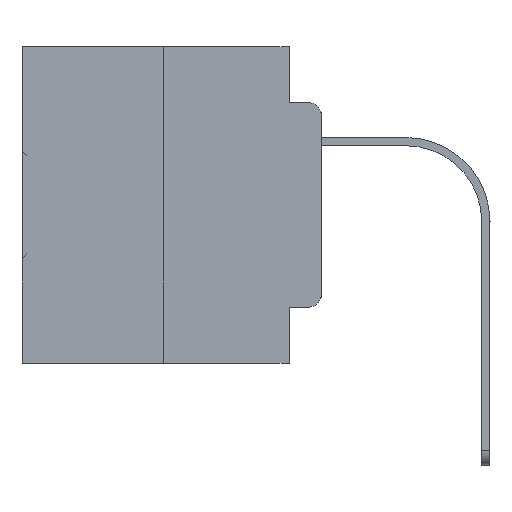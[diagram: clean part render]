
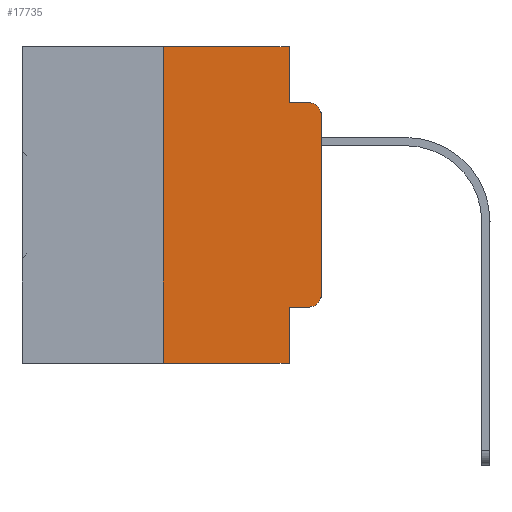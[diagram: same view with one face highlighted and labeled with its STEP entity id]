
A CAD part, left-side view. The second image highlights one B-rep face of the part: STEP entity #17735.
In plain terms, the highlighted planar face has unit normal (-1, 0, 0).
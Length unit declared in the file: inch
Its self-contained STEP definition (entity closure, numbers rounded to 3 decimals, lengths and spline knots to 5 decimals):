
#72 = ORIENTED_EDGE ( 'NONE', *, *, #4562, .T. ) ;
#617 = EDGE_CURVE ( 'NONE', #17997, #18075, #26563, .T. ) ;
#874 = LINE ( 'NONE', #11396, #5345 ) ;
#1128 = AXIS2_PLACEMENT_3D ( 'NONE', #1183, #4248, #24849 ) ;
#1183 = CARTESIAN_POINT ( 'NONE',  ( 0., 0.473, 0. ) ) ;
#2091 = ORIENTED_EDGE ( 'NONE', *, *, #3059, .T. ) ;
#2122 = VECTOR ( 'NONE', #11495, 39.37008 ) ;
#2495 = DIRECTION ( 'NONE',  ( 0., 0., -1. ) ) ;
#2520 = DIRECTION ( 'NONE',  ( 0., -1., 0. ) ) ;
#2718 = ORIENTED_EDGE ( 'NONE', *, *, #12810, .F. ) ;
#2792 = VERTEX_POINT ( 'NONE', #27688 ) ;
#2999 = VERTEX_POINT ( 'NONE', #15572 ) ;
#3022 = LINE ( 'NONE', #28552, #10541 ) ;
#3059 = EDGE_CURVE ( 'NONE', #33369, #26670, #8755, .T. ) ;
#3613 = VERTEX_POINT ( 'NONE', #24059 ) ;
#3626 = DIRECTION ( 'NONE',  ( 0., 0., -1. ) ) ;
#4248 = DIRECTION ( 'NONE',  ( 1., 0., 0. ) ) ;
#4319 = EDGE_CURVE ( 'NONE', #26670, #29849, #8760, .T. ) ;
#4562 = EDGE_CURVE ( 'NONE', #29849, #11041, #17282, .T. ) ;
#5345 = VECTOR ( 'NONE', #11224, 39.37008 ) ;
#6032 = LINE ( 'NONE', #13693, #25964 ) ;
#6205 = DIRECTION ( 'NONE',  ( 0., -1., 0. ) ) ;
#6597 = ORIENTED_EDGE ( 'NONE', *, *, #16310, .F. ) ;
#6738 = LINE ( 'NONE', #19530, #2122 ) ;
#7022 = EDGE_CURVE ( 'NONE', #27252, #17997, #3022, .T. ) ;
#7392 = ORIENTED_EDGE ( 'NONE', *, *, #4319, .T. ) ;
#7935 = EDGE_LOOP ( 'NONE', ( #72, #23176, #6597, #8799, #8987, #2718, #33330, #25415, #2091, #7392 ) ) ;
#8415 = DIRECTION ( 'NONE',  ( 0., -1., 0. ) ) ;
#8755 = LINE ( 'NONE', #23934, #25609 ) ;
#8760 = CIRCLE ( 'NONE', #31046, 0.02 ) ;
#8799 = ORIENTED_EDGE ( 'NONE', *, *, #617, .F. ) ;
#8987 = ORIENTED_EDGE ( 'NONE', *, *, #7022, .F. ) ;
#9286 = EDGE_CURVE ( 'NONE', #11041, #2999, #29083, .T. ) ;
#10429 = CARTESIAN_POINT ( 'NONE',  ( 0., 0.051, -0.4115 ) ) ;
#10541 = VECTOR ( 'NONE', #2520, 39.37008 ) ;
#10921 = DIRECTION ( 'NONE',  ( -1., 0., 0. ) ) ;
#11041 = VERTEX_POINT ( 'NONE', #16896 ) ;
#11224 = DIRECTION ( 'NONE',  ( 0., 0., 1. ) ) ;
#11269 = CARTESIAN_POINT ( 'NONE',  ( 0., 0.02, -0.1085 ) ) ;
#11396 = CARTESIAN_POINT ( 'NONE',  ( 0., 0.25, 0. ) ) ;
#11495 = DIRECTION ( 'NONE',  ( 0., -1., 0. ) ) ;
#11894 = CARTESIAN_POINT ( 'NONE',  ( 0., 0., -0.3915 ) ) ;
#12717 = EDGE_CURVE ( 'NONE', #33369, #2792, #25888, .T. ) ;
#12810 = EDGE_CURVE ( 'NONE', #3613, #27252, #874, .T. ) ;
#13277 = DIRECTION ( 'NONE',  ( 0., 0., -1. ) ) ;
#13562 = CARTESIAN_POINT ( 'NONE',  ( 0., 0.051, -0.0885 ) ) ;
#13693 = CARTESIAN_POINT ( 'NONE',  ( 0., 0.473, -0.5 ) ) ;
#15417 = CARTESIAN_POINT ( 'NONE',  ( 0., 0.02, -0.3915 ) ) ;
#15572 = CARTESIAN_POINT ( 'NONE',  ( 0., 0.02, -0.0885 ) ) ;
#16310 = EDGE_CURVE ( 'NONE', #18075, #2999, #6738, .T. ) ;
#16789 = VECTOR ( 'NONE', #33542, 39.37008 ) ;
#16896 = CARTESIAN_POINT ( 'NONE',  ( 0., 0., -0.1085 ) ) ;
#16965 = CARTESIAN_POINT ( 'NONE',  ( 0., 0.25, 0. ) ) ;
#17282 = LINE ( 'NONE', #27330, #19696 ) ;
#17607 = DIRECTION ( 'NONE',  ( 0., 0., 1. ) ) ;
#17735 = ADVANCED_FACE ( 'NONE', ( #27055 ), #24501, .F. ) ;
#17997 = VERTEX_POINT ( 'NONE', #31449 ) ;
#18075 = VERTEX_POINT ( 'NONE', #13562 ) ;
#19530 = CARTESIAN_POINT ( 'NONE',  ( 0., 0.051, -0.0885 ) ) ;
#19696 = VECTOR ( 'NONE', #17607, 39.37008 ) ;
#21145 = EDGE_CURVE ( 'NONE', #3613, #2792, #6032, .T. ) ;
#23167 = CARTESIAN_POINT ( 'NONE',  ( 0., 0.051, 0. ) ) ;
#23176 = ORIENTED_EDGE ( 'NONE', *, *, #9286, .T. ) ;
#23934 = CARTESIAN_POINT ( 'NONE',  ( 0., 0.051, -0.4115 ) ) ;
#24059 = CARTESIAN_POINT ( 'NONE',  ( 0., 0.25, -0.5 ) ) ;
#24501 = PLANE ( 'NONE',  #1128 ) ;
#24849 = DIRECTION ( 'NONE',  ( 0., 0., -1. ) ) ;
#25281 = AXIS2_PLACEMENT_3D ( 'NONE', #11269, #10921, #3626 ) ;
#25303 = CARTESIAN_POINT ( 'NONE',  ( 0., 0.02, -0.4115 ) ) ;
#25415 = ORIENTED_EDGE ( 'NONE', *, *, #12717, .F. ) ;
#25609 = VECTOR ( 'NONE', #8415, 39.37008 ) ;
#25809 = DIRECTION ( 'NONE',  ( -1., 0., 0. ) ) ;
#25888 = LINE ( 'NONE', #23167, #16789 ) ;
#25964 = VECTOR ( 'NONE', #6205, 39.37008 ) ;
#26054 = CARTESIAN_POINT ( 'NONE',  ( 0., 0.051, 0. ) ) ;
#26563 = LINE ( 'NONE', #26054, #28800 ) ;
#26670 = VERTEX_POINT ( 'NONE', #25303 ) ;
#27055 = FACE_OUTER_BOUND ( 'NONE', #7935, .T. ) ;
#27252 = VERTEX_POINT ( 'NONE', #16965 ) ;
#27330 = CARTESIAN_POINT ( 'NONE',  ( 0., 0., 0. ) ) ;
#27688 = CARTESIAN_POINT ( 'NONE',  ( 0., 0.051, -0.5 ) ) ;
#28552 = CARTESIAN_POINT ( 'NONE',  ( 0., 0.473, 0. ) ) ;
#28800 = VECTOR ( 'NONE', #13277, 39.37008 ) ;
#29083 = CIRCLE ( 'NONE', #25281, 0.02 ) ;
#29849 = VERTEX_POINT ( 'NONE', #11894 ) ;
#31046 = AXIS2_PLACEMENT_3D ( 'NONE', #15417, #25809, #2495 ) ;
#31449 = CARTESIAN_POINT ( 'NONE',  ( 0., 0.051, 0. ) ) ;
#33330 = ORIENTED_EDGE ( 'NONE', *, *, #21145, .T. ) ;
#33369 = VERTEX_POINT ( 'NONE', #10429 ) ;
#33542 = DIRECTION ( 'NONE',  ( 0., 0., -1. ) ) ;
